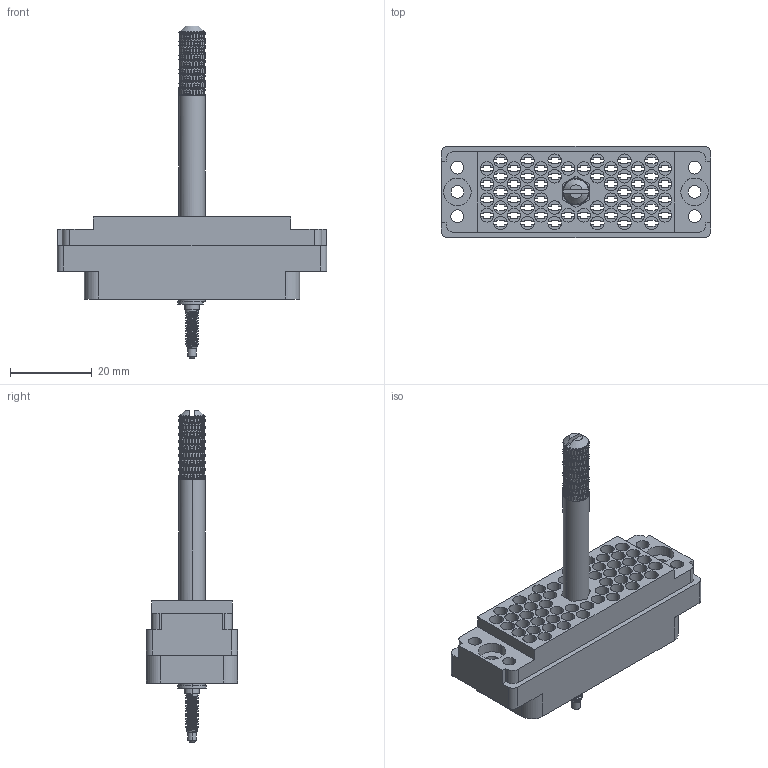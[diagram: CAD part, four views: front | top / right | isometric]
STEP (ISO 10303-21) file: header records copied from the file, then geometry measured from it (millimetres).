
FILE_DESCRIPTION (( 'STEP AP203' ), '1' );
FILE_NAME ('516-056-000-305.STEP', '2020-03-10T04:24:42', ( '' ), ( '' ), 'SwSTEP 2.0', 'SolidWorks 2016', '' );
FILE_SCHEMA (( 'CONFIG_CONTROL_DESIGN' ));
Length unit declared in the file: inch
Products named in the file (7): 516-253-035-100; Actuating Screw Assy 038-056; 516-251-035-100; 516-253-138-107; 516-250-038-111; 516 Plug Insulator_056; 516-056-000-305
Assembly tree (7 placements, depth 3):
  516-056-000-305
    516 Plug Insulator_056
    Actuating Screw Assy 038-056
      516-251-035-100
      516-253-035-100  x2
      516-253-138-107
      516-250-038-111
Bounding box: 65.81 x 22.25 x 81.03 mm (x, y, z)
Volume: 13219.7 mm3; surface area: 17269.5 mm2
Topology: 6 solids, 6 shells, 2618 faces, 6596 edges, 4010 vertices
Faces by surface type: bspline 1006, plane 973, cylinder 619, cone 20
Entity records: 107842 total; most frequent: CARTESIAN_POINT 55372, ORIENTED_EDGE 13168, DIRECTION 8205, EDGE_CURVE 6584, VERTEX_POINT 4002, VECTOR 2851, LINE 2851, EDGE_LOOP 2762
